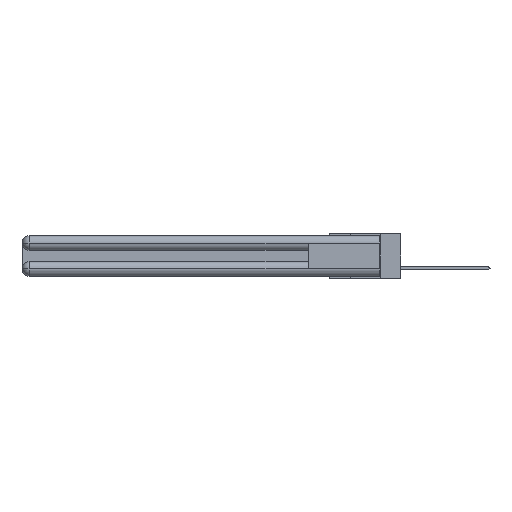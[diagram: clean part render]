
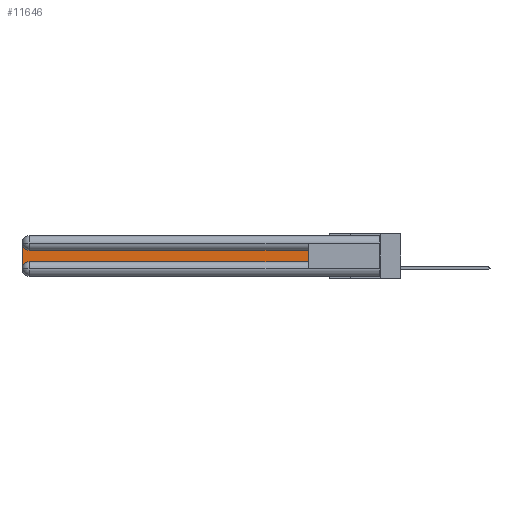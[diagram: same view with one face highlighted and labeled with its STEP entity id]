
A CAD part, left-side view. The second image highlights one B-rep face of the part: STEP entity #11646.
In plain terms, the highlighted planar face has unit normal (-1, 0, 0).
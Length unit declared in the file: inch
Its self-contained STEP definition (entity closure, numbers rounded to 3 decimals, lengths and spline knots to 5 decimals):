
#122 = LINE ( 'NONE', #993, #9290 ) ;
#900 = CARTESIAN_POINT ( 'NONE',  ( 0.075, 3., -0.0625 ) ) ;
#993 = CARTESIAN_POINT ( 'NONE',  ( 0.075, 0.6, -0.1225 ) ) ;
#1701 = EDGE_CURVE ( 'NONE', #17526, #3608, #11670, .T. ) ;
#1905 = DIRECTION ( 'NONE',  ( 0., 0., -1. ) ) ;
#2160 = VECTOR ( 'NONE', #13928, 39.37008 ) ;
#3608 = VERTEX_POINT ( 'NONE', #20933 ) ;
#5267 = ORIENTED_EDGE ( 'NONE', *, *, #27826, .T. ) ;
#5311 = ORIENTED_EDGE ( 'NONE', *, *, #11042, .T. ) ;
#6627 = VERTEX_POINT ( 'NONE', #24218 ) ;
#6660 = ORIENTED_EDGE ( 'NONE', *, *, #7104, .T. ) ;
#7104 = EDGE_CURVE ( 'NONE', #7764, #17526, #19829, .T. ) ;
#7323 = DIRECTION ( 'NONE',  ( 0., -1., 0. ) ) ;
#7416 = DIRECTION ( 'NONE',  ( 0., 0., -1. ) ) ;
#7764 = VERTEX_POINT ( 'NONE', #13085 ) ;
#8334 = EDGE_CURVE ( 'NONE', #9892, #18200, #19195, .T. ) ;
#8526 = CARTESIAN_POINT ( 'NONE',  ( 0.075, 2.94, -0.1225 ) ) ;
#9180 = EDGE_LOOP ( 'NONE', ( #5267, #25752, #12347, #6660, #19554, #5311 ) ) ;
#9290 = VECTOR ( 'NONE', #27857, 39.37008 ) ;
#9413 = CARTESIAN_POINT ( 'NONE',  ( 0.075, 0.6, -0.2175 ) ) ;
#9423 = AXIS2_PLACEMENT_3D ( 'NONE', #10468, #15174, #1905 ) ;
#9892 = VERTEX_POINT ( 'NONE', #8526 ) ;
#10282 = LINE ( 'NONE', #9413, #2160 ) ;
#10468 = CARTESIAN_POINT ( 'NONE',  ( 0.075, 2.94, -0.2775 ) ) ;
#11042 = EDGE_CURVE ( 'NONE', #3608, #6627, #10282, .T. ) ;
#11646 = ADVANCED_FACE ( 'NONE', ( #22435 ), #23399, .F. ) ;
#11670 = LINE ( 'NONE', #22399, #18226 ) ;
#12159 = AXIS2_PLACEMENT_3D ( 'NONE', #21040, #25635, #16645 ) ;
#12347 = ORIENTED_EDGE ( 'NONE', *, *, #21853, .T. ) ;
#12675 = AXIS2_PLACEMENT_3D ( 'NONE', #18671, #27483, #7416 ) ;
#13085 = CARTESIAN_POINT ( 'NONE',  ( 0.075, 3., -0.2775 ) ) ;
#13928 = DIRECTION ( 'NONE',  ( 0., 0., 1. ) ) ;
#15174 = DIRECTION ( 'NONE',  ( 1., 0., 0. ) ) ;
#16347 = CARTESIAN_POINT ( 'NONE',  ( 0.075, 2.94, -0.2175 ) ) ;
#16645 = DIRECTION ( 'NONE',  ( 0., 0., -1. ) ) ;
#17526 = VERTEX_POINT ( 'NONE', #16347 ) ;
#18200 = VERTEX_POINT ( 'NONE', #900 ) ;
#18226 = VECTOR ( 'NONE', #7323, 39.37008 ) ;
#18671 = CARTESIAN_POINT ( 'NONE',  ( 0.075, 2.94, -0.0625 ) ) ;
#19195 = CIRCLE ( 'NONE', #12675, 0.06 ) ;
#19554 = ORIENTED_EDGE ( 'NONE', *, *, #1701, .T. ) ;
#19829 = CIRCLE ( 'NONE', #9423, 0.06 ) ;
#20933 = CARTESIAN_POINT ( 'NONE',  ( 0.075, 0.6, -0.2175 ) ) ;
#21040 = CARTESIAN_POINT ( 'NONE',  ( 0.075, 3., -0.1225 ) ) ;
#21853 = EDGE_CURVE ( 'NONE', #18200, #7764, #29011, .T. ) ;
#22399 = CARTESIAN_POINT ( 'NONE',  ( 0.075, 0.6, -0.2175 ) ) ;
#22435 = FACE_OUTER_BOUND ( 'NONE', #9180, .T. ) ;
#23399 = PLANE ( 'NONE',  #12159 ) ;
#24089 = VECTOR ( 'NONE', #28817, 39.37008 ) ;
#24218 = CARTESIAN_POINT ( 'NONE',  ( 0.075, 0.6, -0.1225 ) ) ;
#24294 = CARTESIAN_POINT ( 'NONE',  ( 0.075, 3., -0.2175 ) ) ;
#25635 = DIRECTION ( 'NONE',  ( 1., 0., 0. ) ) ;
#25752 = ORIENTED_EDGE ( 'NONE', *, *, #8334, .T. ) ;
#27483 = DIRECTION ( 'NONE',  ( 1., 0., 0. ) ) ;
#27826 = EDGE_CURVE ( 'NONE', #6627, #9892, #122, .T. ) ;
#27857 = DIRECTION ( 'NONE',  ( 0., 1., 0. ) ) ;
#28817 = DIRECTION ( 'NONE',  ( 0., 0., -1. ) ) ;
#29011 = LINE ( 'NONE', #24294, #24089 ) ;
